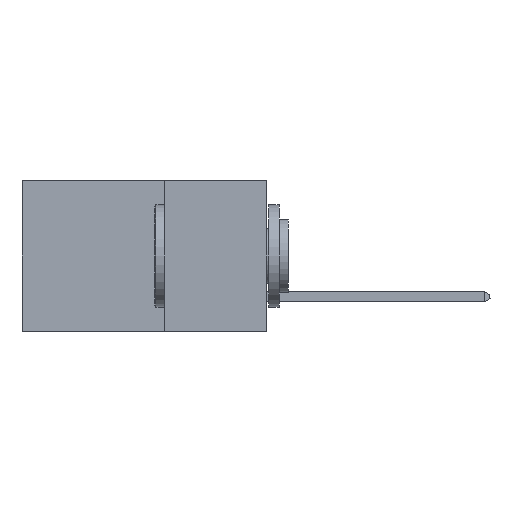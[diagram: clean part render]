
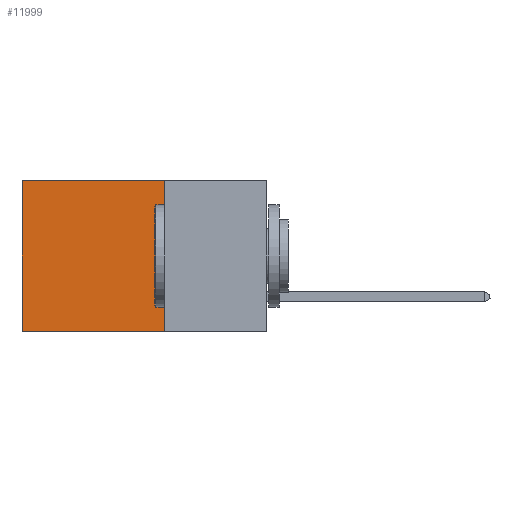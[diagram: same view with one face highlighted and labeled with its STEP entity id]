
A CAD part, left-side view. The second image highlights one B-rep face of the part: STEP entity #11999.
In plain terms, the highlighted planar face has unit normal (-1, 0, 0).
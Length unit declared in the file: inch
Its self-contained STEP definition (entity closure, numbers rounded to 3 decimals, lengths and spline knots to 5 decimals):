
#120 = ORIENTED_EDGE ( 'NONE', *, *, #9291, .T. ) ;
#697 = CARTESIAN_POINT ( 'NONE',  ( 0.2875, 0.25, -0.37 ) ) ;
#726 = FACE_OUTER_BOUND ( 'NONE', #6445, .T. ) ;
#804 = DIRECTION ( 'NONE',  ( 1., 0., 0. ) ) ;
#910 = VECTOR ( 'NONE', #9670, 39.37008 ) ;
#975 = VERTEX_POINT ( 'NONE', #3284 ) ;
#1200 = CARTESIAN_POINT ( 'NONE',  ( 0.2875, 0.25, 0. ) ) ;
#1529 = EDGE_CURVE ( 'NONE', #10225, #3664, #2934, .T. ) ;
#1621 = DIRECTION ( 'NONE',  ( 0., 0., -1. ) ) ;
#1663 = CARTESIAN_POINT ( 'NONE',  ( 0.2875, 0.25, 0. ) ) ;
#2160 = DIRECTION ( 'NONE',  ( 0., 1., 0. ) ) ;
#2398 = VECTOR ( 'NONE', #9576, 39.37008 ) ;
#2855 = ORIENTED_EDGE ( 'NONE', *, *, #9122, .T. ) ;
#2934 = LINE ( 'NONE', #697, #6229 ) ;
#3012 = VECTOR ( 'NONE', #2160, 39.37008 ) ;
#3079 = CARTESIAN_POINT ( 'NONE',  ( 0.2875, 0.25, 0. ) ) ;
#3107 = CARTESIAN_POINT ( 'NONE',  ( 0.2875, 0.25, -0.37 ) ) ;
#3284 = CARTESIAN_POINT ( 'NONE',  ( 0.2875, 0.25, 0. ) ) ;
#3664 = VERTEX_POINT ( 'NONE', #6294 ) ;
#3848 = CARTESIAN_POINT ( 'NONE',  ( 0.2875, 0.6, 0. ) ) ;
#4975 = LINE ( 'NONE', #3848, #2398 ) ;
#5493 = ORIENTED_EDGE ( 'NONE', *, *, #11522, .F. ) ;
#5579 = DIRECTION ( 'NONE',  ( 0., 1., 0. ) ) ;
#5764 = LINE ( 'NONE', #3079, #910 ) ;
#6229 = VECTOR ( 'NONE', #5579, 39.37008 ) ;
#6294 = CARTESIAN_POINT ( 'NONE',  ( 0.2875, 0.6, -0.37 ) ) ;
#6445 = EDGE_LOOP ( 'NONE', ( #120, #9764, #5493, #2855 ) ) ;
#6612 = CARTESIAN_POINT ( 'NONE',  ( 0.2875, 0.6, 0. ) ) ;
#7427 = PLANE ( 'NONE',  #12489 ) ;
#8758 = LINE ( 'NONE', #1200, #3012 ) ;
#9122 = EDGE_CURVE ( 'NONE', #975, #9286, #8758, .T. ) ;
#9286 = VERTEX_POINT ( 'NONE', #6612 ) ;
#9291 = EDGE_CURVE ( 'NONE', #9286, #3664, #4975, .T. ) ;
#9576 = DIRECTION ( 'NONE',  ( 0., 0., -1. ) ) ;
#9670 = DIRECTION ( 'NONE',  ( 0., 0., -1. ) ) ;
#9764 = ORIENTED_EDGE ( 'NONE', *, *, #1529, .F. ) ;
#10225 = VERTEX_POINT ( 'NONE', #3107 ) ;
#11522 = EDGE_CURVE ( 'NONE', #975, #10225, #5764, .T. ) ;
#11999 = ADVANCED_FACE ( 'NONE', ( #726 ), #7427, .F. ) ;
#12489 = AXIS2_PLACEMENT_3D ( 'NONE', #1663, #804, #1621 ) ;
